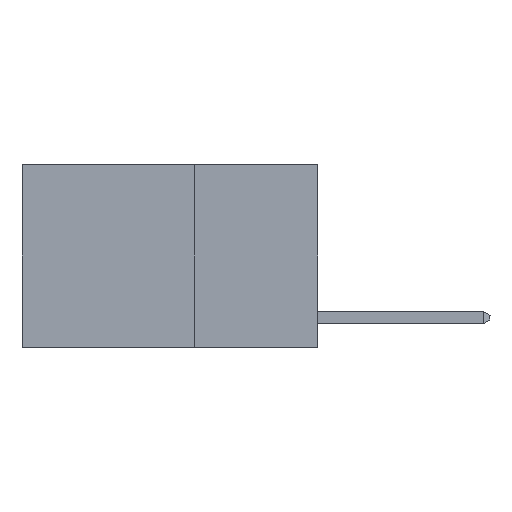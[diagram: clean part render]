
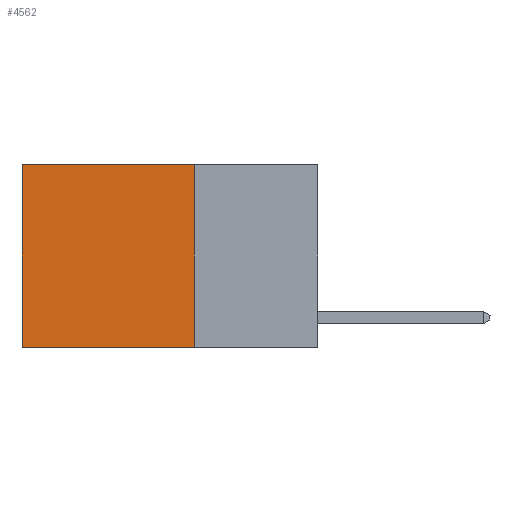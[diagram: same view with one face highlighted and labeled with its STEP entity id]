
A CAD part, left-side view. The second image highlights one B-rep face of the part: STEP entity #4562.
In plain terms, the highlighted planar face has unit normal (-1, 0, 0).
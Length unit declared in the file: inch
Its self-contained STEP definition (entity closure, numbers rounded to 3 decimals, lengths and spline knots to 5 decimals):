
#126 = VERTEX_POINT ( 'NONE', #11887 ) ;
#384 = ORIENTED_EDGE ( 'NONE', *, *, #17846, .T. ) ;
#716 = DIRECTION ( 'NONE',  ( 0., 1., 0. ) ) ;
#1497 = VECTOR ( 'NONE', #1939, 39.37008 ) ;
#1939 = DIRECTION ( 'NONE',  ( 0., 0., -1. ) ) ;
#2573 = VERTEX_POINT ( 'NONE', #3169 ) ;
#3039 = DIRECTION ( 'NONE',  ( 0., 0., -1. ) ) ;
#3169 = CARTESIAN_POINT ( 'NONE',  ( 0.2625, 0.25, -0.37 ) ) ;
#3542 = LINE ( 'NONE', #17766, #1497 ) ;
#3634 = LINE ( 'NONE', #9080, #12276 ) ;
#4419 = ORIENTED_EDGE ( 'NONE', *, *, #10588, .T. ) ;
#4562 = ADVANCED_FACE ( 'NONE', ( #8420 ), #9894, .F. ) ;
#5536 = CARTESIAN_POINT ( 'NONE',  ( 0.2625, 0.25, 0. ) ) ;
#5677 = EDGE_CURVE ( 'NONE', #12248, #2573, #3634, .T. ) ;
#6974 = CARTESIAN_POINT ( 'NONE',  ( 0.2625, 0.25, -0.37 ) ) ;
#7058 = DIRECTION ( 'NONE',  ( 0., 1., 0. ) ) ;
#7556 = VECTOR ( 'NONE', #716, 39.37008 ) ;
#7578 = ORIENTED_EDGE ( 'NONE', *, *, #17607, .F. ) ;
#8011 = VECTOR ( 'NONE', #7058, 39.37008 ) ;
#8420 = FACE_OUTER_BOUND ( 'NONE', #16554, .T. ) ;
#9080 = CARTESIAN_POINT ( 'NONE',  ( 0.2625, 0.25, 0. ) ) ;
#9163 = CARTESIAN_POINT ( 'NONE',  ( 0.2625, 0.25, 0. ) ) ;
#9894 = PLANE ( 'NONE',  #16938 ) ;
#10588 = EDGE_CURVE ( 'NONE', #12248, #14857, #14703, .T. ) ;
#11133 = LINE ( 'NONE', #6974, #8011 ) ;
#11732 = CARTESIAN_POINT ( 'NONE',  ( 0.2625, 0.25, 0. ) ) ;
#11887 = CARTESIAN_POINT ( 'NONE',  ( 0.2625, 0.6, -0.37 ) ) ;
#12248 = VERTEX_POINT ( 'NONE', #11732 ) ;
#12276 = VECTOR ( 'NONE', #17491, 39.37008 ) ;
#14703 = LINE ( 'NONE', #9163, #7556 ) ;
#14857 = VERTEX_POINT ( 'NONE', #15937 ) ;
#15697 = DIRECTION ( 'NONE',  ( 1., 0., 0. ) ) ;
#15937 = CARTESIAN_POINT ( 'NONE',  ( 0.2625, 0.6, 0. ) ) ;
#16554 = EDGE_LOOP ( 'NONE', ( #384, #7578, #17924, #4419 ) ) ;
#16938 = AXIS2_PLACEMENT_3D ( 'NONE', #5536, #15697, #3039 ) ;
#17491 = DIRECTION ( 'NONE',  ( 0., 0., -1. ) ) ;
#17607 = EDGE_CURVE ( 'NONE', #2573, #126, #11133, .T. ) ;
#17766 = CARTESIAN_POINT ( 'NONE',  ( 0.2625, 0.6, 0. ) ) ;
#17846 = EDGE_CURVE ( 'NONE', #14857, #126, #3542, .T. ) ;
#17924 = ORIENTED_EDGE ( 'NONE', *, *, #5677, .F. ) ;
